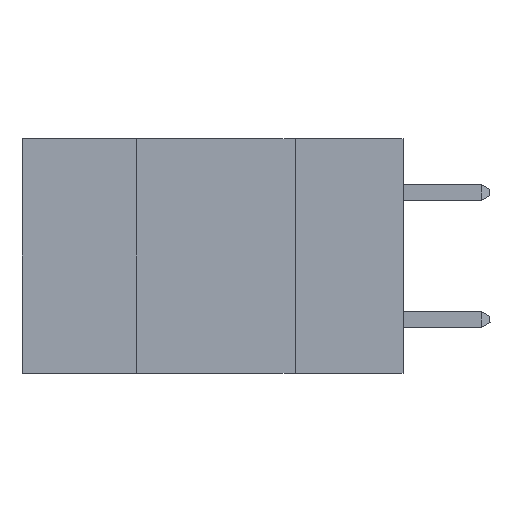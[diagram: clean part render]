
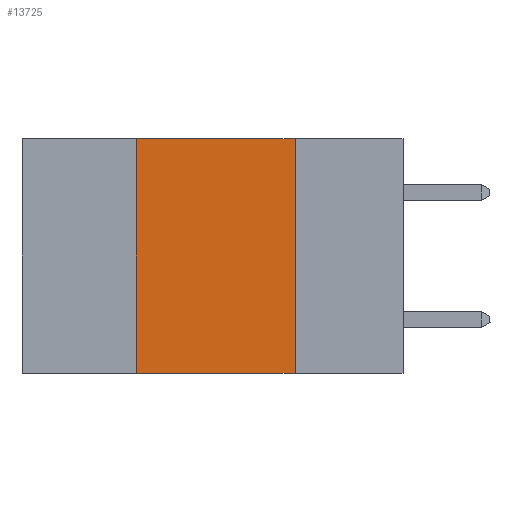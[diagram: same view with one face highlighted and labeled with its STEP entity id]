
A CAD part, left-side view. The second image highlights one B-rep face of the part: STEP entity #13725.
In plain terms, the highlighted planar face has unit normal (-1, 0, 0).
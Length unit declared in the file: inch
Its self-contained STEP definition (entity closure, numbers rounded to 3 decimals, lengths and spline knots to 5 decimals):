
#28 = LINE ( 'NONE', #9995, #11660 ) ;
#126 = EDGE_CURVE ( 'NONE', #5606, #13219, #15380, .T. ) ;
#359 = ORIENTED_EDGE ( 'NONE', *, *, #1255, .F. ) ;
#900 = DIRECTION ( 'NONE',  ( 0., 0., -1. ) ) ;
#1255 = EDGE_CURVE ( 'NONE', #5606, #2933, #5722, .T. ) ;
#1417 = AXIS2_PLACEMENT_3D ( 'NONE', #2896, #3198, #900 ) ;
#1708 = PLANE ( 'NONE',  #1417 ) ;
#1724 = ORIENTED_EDGE ( 'NONE', *, *, #4130, .F. ) ;
#2896 = CARTESIAN_POINT ( 'NONE',  ( 0., 0.6, 0. ) ) ;
#2933 = VERTEX_POINT ( 'NONE', #9548 ) ;
#3198 = DIRECTION ( 'NONE',  ( 1., 0., 0. ) ) ;
#3615 = ORIENTED_EDGE ( 'NONE', *, *, #126, .T. ) ;
#4130 = EDGE_CURVE ( 'NONE', #2933, #6702, #11303, .T. ) ;
#4229 = DIRECTION ( 'NONE',  ( 0., -1., 0. ) ) ;
#4391 = DIRECTION ( 'NONE',  ( 0., 0., 1. ) ) ;
#4528 = DIRECTION ( 'NONE',  ( 0., 0., -1. ) ) ;
#5606 = VERTEX_POINT ( 'NONE', #7210 ) ;
#5664 = EDGE_LOOP ( 'NONE', ( #9466, #1724, #359, #3615 ) ) ;
#5722 = LINE ( 'NONE', #6445, #14944 ) ;
#5952 = VECTOR ( 'NONE', #9214, 39.37008 ) ;
#6445 = CARTESIAN_POINT ( 'NONE',  ( 0., 0.42, 0. ) ) ;
#6702 = VERTEX_POINT ( 'NONE', #9018 ) ;
#7210 = CARTESIAN_POINT ( 'NONE',  ( 0., 0.42, -0.37 ) ) ;
#8111 = VECTOR ( 'NONE', #4229, 39.37008 ) ;
#9018 = CARTESIAN_POINT ( 'NONE',  ( 0., 0.17, 0. ) ) ;
#9214 = DIRECTION ( 'NONE',  ( 0., -1., 0. ) ) ;
#9466 = ORIENTED_EDGE ( 'NONE', *, *, #13570, .F. ) ;
#9485 = CARTESIAN_POINT ( 'NONE',  ( 0., 0.17, -0.37 ) ) ;
#9548 = CARTESIAN_POINT ( 'NONE',  ( 0., 0.42, 0. ) ) ;
#9995 = CARTESIAN_POINT ( 'NONE',  ( 0., 0.17, 0. ) ) ;
#11303 = LINE ( 'NONE', #14713, #8111 ) ;
#11660 = VECTOR ( 'NONE', #4528, 39.37008 ) ;
#12596 = FACE_OUTER_BOUND ( 'NONE', #5664, .T. ) ;
#13219 = VERTEX_POINT ( 'NONE', #9485 ) ;
#13570 = EDGE_CURVE ( 'NONE', #6702, #13219, #28, .T. ) ;
#13725 = ADVANCED_FACE ( 'NONE', ( #12596 ), #1708, .F. ) ;
#13850 = CARTESIAN_POINT ( 'NONE',  ( 0., 0.6, -0.37 ) ) ;
#14713 = CARTESIAN_POINT ( 'NONE',  ( 0., 0.6, 0. ) ) ;
#14944 = VECTOR ( 'NONE', #4391, 39.37008 ) ;
#15380 = LINE ( 'NONE', #13850, #5952 ) ;
